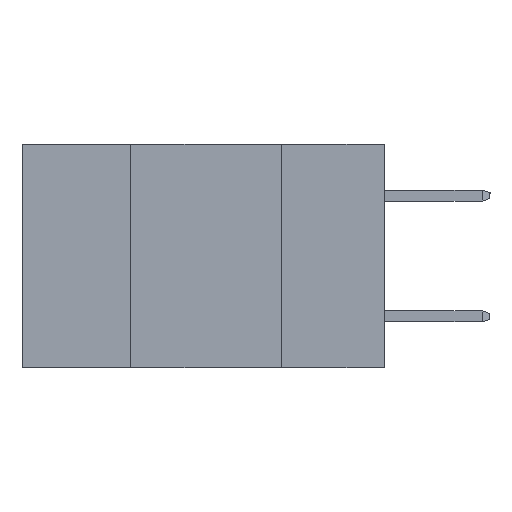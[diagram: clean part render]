
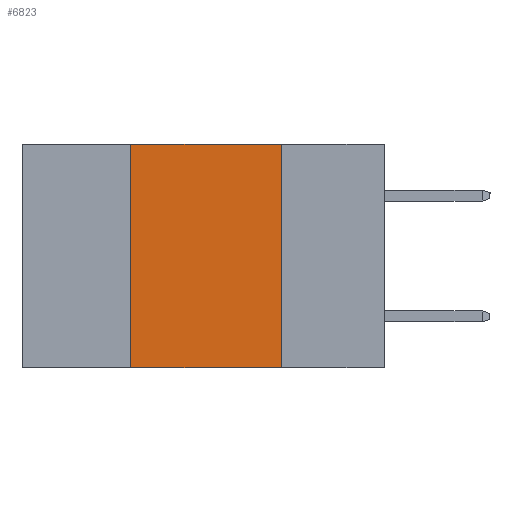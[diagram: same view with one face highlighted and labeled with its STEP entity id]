
A CAD part, left-side view. The second image highlights one B-rep face of the part: STEP entity #6823.
In plain terms, the highlighted planar face has unit normal (-1, 0, 0).
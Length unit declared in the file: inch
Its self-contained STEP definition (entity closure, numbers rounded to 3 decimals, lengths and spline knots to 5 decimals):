
#38 = CARTESIAN_POINT ( 'NONE',  ( 0., 0.42, -0.37 ) ) ;
#3533 = FACE_OUTER_BOUND ( 'NONE', #9367, .T. ) ;
#3574 = DIRECTION ( 'NONE',  ( 0., -1., 0. ) ) ;
#3807 = LINE ( 'NONE', #14067, #20100 ) ;
#4160 = EDGE_CURVE ( 'NONE', #18581, #11576, #3807, .T. ) ;
#5138 = ORIENTED_EDGE ( 'NONE', *, *, #15928, .T. ) ;
#5374 = ORIENTED_EDGE ( 'NONE', *, *, #13096, .F. ) ;
#6004 = ORIENTED_EDGE ( 'NONE', *, *, #17117, .F. ) ;
#6097 = DIRECTION ( 'NONE',  ( 0., 0., -1. ) ) ;
#6686 = DIRECTION ( 'NONE',  ( 1., 0., 0. ) ) ;
#6823 = ADVANCED_FACE ( 'NONE', ( #3533 ), #15216, .F. ) ;
#6838 = CARTESIAN_POINT ( 'NONE',  ( 0., 0.6, -0.37 ) ) ;
#7629 = CARTESIAN_POINT ( 'NONE',  ( 0., 0.17, -0.37 ) ) ;
#9367 = EDGE_LOOP ( 'NONE', ( #6004, #10715, #5374, #5138 ) ) ;
#9656 = VERTEX_POINT ( 'NONE', #38 ) ;
#9714 = VECTOR ( 'NONE', #13920, 39.37008 ) ;
#9786 = LINE ( 'NONE', #6838, #16801 ) ;
#10181 = DIRECTION ( 'NONE',  ( 0., 0., -1. ) ) ;
#10715 = ORIENTED_EDGE ( 'NONE', *, *, #4160, .F. ) ;
#11576 = VERTEX_POINT ( 'NONE', #13761 ) ;
#13096 = EDGE_CURVE ( 'NONE', #9656, #18581, #20738, .T. ) ;
#13761 = CARTESIAN_POINT ( 'NONE',  ( 0., 0.17, 0. ) ) ;
#13920 = DIRECTION ( 'NONE',  ( 0., 0., 1. ) ) ;
#14037 = VECTOR ( 'NONE', #6097, 39.37008 ) ;
#14067 = CARTESIAN_POINT ( 'NONE',  ( 0., 0.6, 0. ) ) ;
#14942 = VERTEX_POINT ( 'NONE', #15247 ) ;
#15216 = PLANE ( 'NONE',  #18635 ) ;
#15247 = CARTESIAN_POINT ( 'NONE',  ( 0., 0.17, -0.37 ) ) ;
#15928 = EDGE_CURVE ( 'NONE', #9656, #14942, #9786, .T. ) ;
#15938 = LINE ( 'NONE', #7629, #14037 ) ;
#16801 = VECTOR ( 'NONE', #3574, 39.37008 ) ;
#17117 = EDGE_CURVE ( 'NONE', #11576, #14942, #15938, .T. ) ;
#17214 = CARTESIAN_POINT ( 'NONE',  ( 0., 0.42, -0.37 ) ) ;
#18000 = CARTESIAN_POINT ( 'NONE',  ( 0., 0.42, 0. ) ) ;
#18581 = VERTEX_POINT ( 'NONE', #18000 ) ;
#18635 = AXIS2_PLACEMENT_3D ( 'NONE', #21472, #6686, #10181 ) ;
#20100 = VECTOR ( 'NONE', #20662, 39.37008 ) ;
#20662 = DIRECTION ( 'NONE',  ( 0., -1., 0. ) ) ;
#20738 = LINE ( 'NONE', #17214, #9714 ) ;
#21472 = CARTESIAN_POINT ( 'NONE',  ( 0., 0.6, 0. ) ) ;
